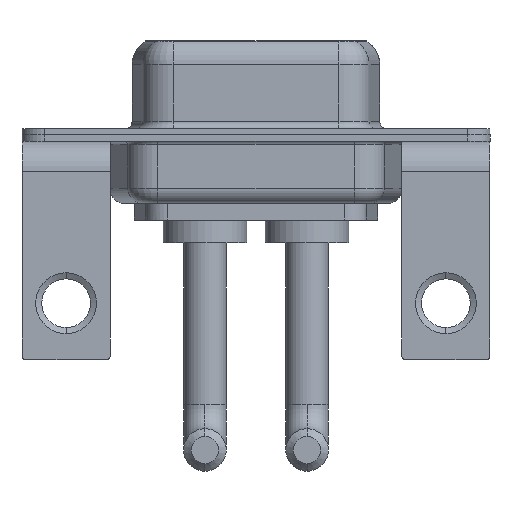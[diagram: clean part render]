
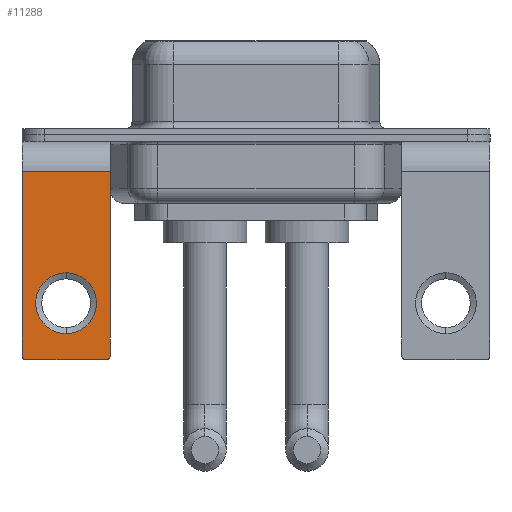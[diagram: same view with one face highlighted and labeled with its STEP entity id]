
A CAD part, front view. The second image highlights one B-rep face of the part: STEP entity #11288.
In plain terms, the highlighted planar face has unit normal (0, -1, 0).
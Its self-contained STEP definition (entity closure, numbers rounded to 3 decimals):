
#115 = VERTEX_POINT ( 'NONE', #11740 ) ;
#192 = DIRECTION ( 'NONE',  ( 0., 1., 0. ) ) ;
#346 = CARTESIAN_POINT ( 'NONE',  ( 2.65, -6.25, -14.8 ) ) ;
#576 = CIRCLE ( 'NONE', #10790, 0.25 ) ;
#963 = VERTEX_POINT ( 'NONE', #5309 ) ;
#1041 = AXIS2_PLACEMENT_3D ( 'NONE', #3747, #5768, #10599 ) ;
#1179 = ORIENTED_EDGE ( 'NONE', *, *, #5530, .T. ) ;
#1298 = EDGE_CURVE ( 'NONE', #2305, #8597, #12798, .T. ) ;
#1563 = CIRCLE ( 'NONE', #7621, 2. ) ;
#1604 = LINE ( 'NONE', #4611, #7078 ) ;
#2159 = FACE_OUTER_BOUND ( 'NONE', #7009, .T. ) ;
#2305 = VERTEX_POINT ( 'NONE', #2777 ) ;
#2652 = EDGE_LOOP ( 'NONE', ( #6486, #7751 ) ) ;
#2711 = VERTEX_POINT ( 'NONE', #4906 ) ;
#2777 = CARTESIAN_POINT ( 'NONE',  ( -2.9, -6.25, -14.55 ) ) ;
#2813 = CARTESIAN_POINT ( 'NONE',  ( -2.65, -6.25, -14.55 ) ) ;
#2818 = VECTOR ( 'NONE', #6103, 1000. ) ;
#3496 = ORIENTED_EDGE ( 'NONE', *, *, #6930, .F. ) ;
#3695 = EDGE_CURVE ( 'NONE', #2711, #10939, #1563, .T. ) ;
#3747 = CARTESIAN_POINT ( 'NONE',  ( 0., -6.25, -11.07 ) ) ;
#3808 = AXIS2_PLACEMENT_3D ( 'NONE', #6068, #192, #5035 ) ;
#3837 = CARTESIAN_POINT ( 'NONE',  ( 2.9, -6.25, -2.4 ) ) ;
#3867 = CARTESIAN_POINT ( 'NONE',  ( 2.65, -6.25, -14.55 ) ) ;
#4563 = ORIENTED_EDGE ( 'NONE', *, *, #4779, .F. ) ;
#4611 = CARTESIAN_POINT ( 'NONE',  ( 2.9, -6.25, -2.4 ) ) ;
#4779 = EDGE_CURVE ( 'NONE', #10801, #8597, #8075, .T. ) ;
#4906 = CARTESIAN_POINT ( 'NONE',  ( 0., -6.25, -9.07 ) ) ;
#5035 = DIRECTION ( 'NONE',  ( 0., 0., 1. ) ) ;
#5309 = CARTESIAN_POINT ( 'NONE',  ( 2.9, -6.25, -14.55 ) ) ;
#5530 = EDGE_CURVE ( 'NONE', #10801, #963, #576, .T. ) ;
#5633 = CIRCLE ( 'NONE', #1041, 2. ) ;
#5768 = DIRECTION ( 'NONE',  ( 0., 1., 0. ) ) ;
#5819 = DIRECTION ( 'NONE',  ( 0., 0., 1. ) ) ;
#6010 = PLANE ( 'NONE',  #3808 ) ;
#6068 = CARTESIAN_POINT ( 'NONE',  ( 2.9, -6.25, -2.4 ) ) ;
#6103 = DIRECTION ( 'NONE',  ( -1., 0., 0. ) ) ;
#6486 = ORIENTED_EDGE ( 'NONE', *, *, #7989, .T. ) ;
#6603 = CARTESIAN_POINT ( 'NONE',  ( -2.65, -6.25, -14.8 ) ) ;
#6781 = DIRECTION ( 'NONE',  ( 0., 0., -1. ) ) ;
#6916 = CARTESIAN_POINT ( 'NONE',  ( 2.9, -6.25, -2.4 ) ) ;
#6930 = EDGE_CURVE ( 'NONE', #6955, #963, #1604, .T. ) ;
#6955 = VERTEX_POINT ( 'NONE', #3837 ) ;
#6966 = CARTESIAN_POINT ( 'NONE',  ( 2.9, -6.25, -14.8 ) ) ;
#7009 = EDGE_LOOP ( 'NONE', ( #8774, #9045, #4563, #1179, #3496, #9941 ) ) ;
#7078 = VECTOR ( 'NONE', #6781, 1000. ) ;
#7165 = CARTESIAN_POINT ( 'NONE',  ( -2.9, -6.25, -2.4 ) ) ;
#7175 = AXIS2_PLACEMENT_3D ( 'NONE', #2813, #10901, #12737 ) ;
#7621 = AXIS2_PLACEMENT_3D ( 'NONE', #8821, #11963, #10844 ) ;
#7751 = ORIENTED_EDGE ( 'NONE', *, *, #3695, .T. ) ;
#7890 = LINE ( 'NONE', #6916, #12142 ) ;
#7989 = EDGE_CURVE ( 'NONE', #10939, #2711, #5633, .T. ) ;
#8025 = DIRECTION ( 'NONE',  ( -1., 0., 0. ) ) ;
#8075 = LINE ( 'NONE', #6966, #2818 ) ;
#8141 = LINE ( 'NONE', #7165, #11969 ) ;
#8597 = VERTEX_POINT ( 'NONE', #6603 ) ;
#8774 = ORIENTED_EDGE ( 'NONE', *, *, #12499, .T. ) ;
#8821 = CARTESIAN_POINT ( 'NONE',  ( 0., -6.25, -11.07 ) ) ;
#9045 = ORIENTED_EDGE ( 'NONE', *, *, #1298, .T. ) ;
#9485 = CARTESIAN_POINT ( 'NONE',  ( 0., -6.25, -13.07 ) ) ;
#9941 = ORIENTED_EDGE ( 'NONE', *, *, #10434, .T. ) ;
#10185 = FACE_BOUND ( 'NONE', #2652, .T. ) ;
#10434 = EDGE_CURVE ( 'NONE', #6955, #115, #7890, .T. ) ;
#10599 = DIRECTION ( 'NONE',  ( 0., 0., 1. ) ) ;
#10790 = AXIS2_PLACEMENT_3D ( 'NONE', #3867, #11696, #5819 ) ;
#10801 = VERTEX_POINT ( 'NONE', #346 ) ;
#10844 = DIRECTION ( 'NONE',  ( 0., 0., 1. ) ) ;
#10901 = DIRECTION ( 'NONE',  ( 0., -1., 0. ) ) ;
#10939 = VERTEX_POINT ( 'NONE', #9485 ) ;
#10949 = DIRECTION ( 'NONE',  ( 0., 0., -1. ) ) ;
#11288 = ADVANCED_FACE ( 'NONE', ( #10185, #2159 ), #6010, .F. ) ;
#11696 = DIRECTION ( 'NONE',  ( 0., -1., 0. ) ) ;
#11740 = CARTESIAN_POINT ( 'NONE',  ( -2.9, -6.25, -2.4 ) ) ;
#11963 = DIRECTION ( 'NONE',  ( 0., 1., 0. ) ) ;
#11969 = VECTOR ( 'NONE', #10949, 1000. ) ;
#12142 = VECTOR ( 'NONE', #8025, 1000. ) ;
#12499 = EDGE_CURVE ( 'NONE', #115, #2305, #8141, .T. ) ;
#12737 = DIRECTION ( 'NONE',  ( 0., 0., 1. ) ) ;
#12798 = CIRCLE ( 'NONE', #7175, 0.25 ) ;
